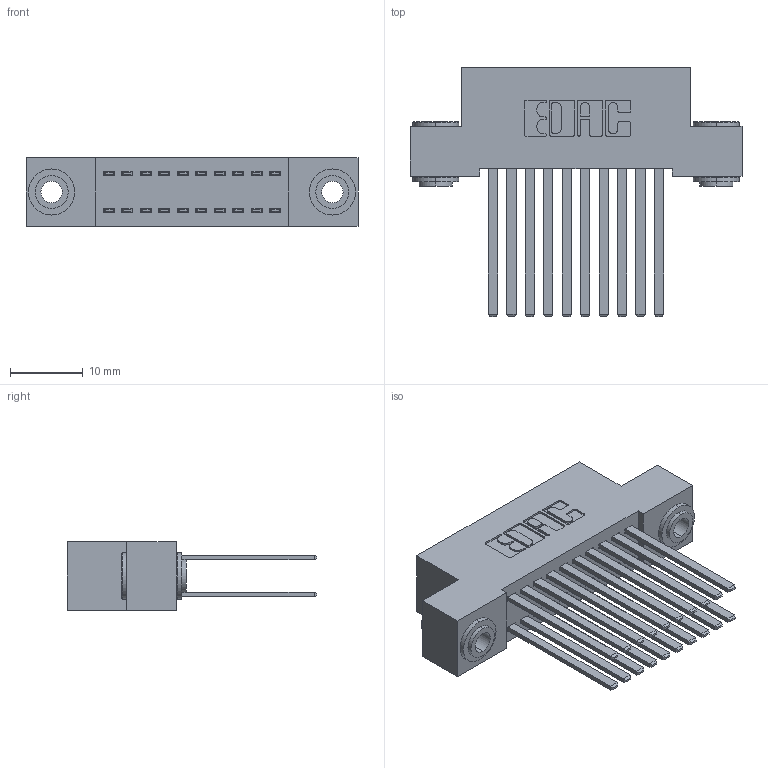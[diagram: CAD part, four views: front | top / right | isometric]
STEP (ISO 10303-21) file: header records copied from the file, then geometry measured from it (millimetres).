
FILE_DESCRIPTION (( 'STEP AP203' ), '1' );
FILE_NAME ('392-020-544-203.STEP', '2019-10-07T05:20:21', ( '' ), ( '' ), 'SwSTEP 2.0', 'SolidWorks 2016', '' );
FILE_SCHEMA (( 'CONFIG_CONTROL_DESIGN' ));
Length unit declared in the file: inch
Products named in the file (4): 345-292-001_345-293-144; 342-250-002_345-250-002-102; 392-020-544-203; 342 Part_.156 TH
Assembly tree (23 placements, depth 2):
  392-020-544-203
    342 Part_.156 TH
    345-292-001_345-293-144  x20
    342-250-002_345-250-002-102  x2
Bounding box: 45.72 x 34.3 x 9.4 mm (x, y, z)
Volume: 4259.7 mm3; surface area: 7135.6 mm2
Topology: 23 solids, 23 shells, 1068 faces, 3115 edges, 2046 vertices
Faces by surface type: plane 716, cylinder 344, cone 8
Entity records: 10906 total; most frequent: CARTESIAN_POINT 1817, ORIENTED_EDGE 1746, DIRECTION 1639, EDGE_CURVE 873, LINE 725, VECTOR 725, VERTEX_POINT 578, AXIS2_PLACEMENT_3D 457
